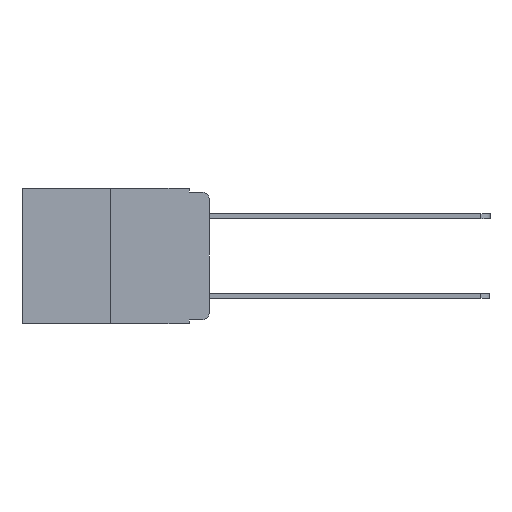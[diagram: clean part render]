
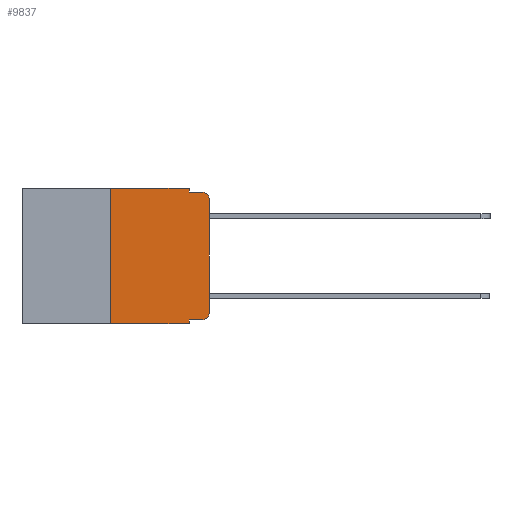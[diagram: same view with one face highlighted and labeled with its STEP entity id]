
A CAD part, left-side view. The second image highlights one B-rep face of the part: STEP entity #9837.
In plain terms, the highlighted planar face has unit normal (-1, 0, 0).
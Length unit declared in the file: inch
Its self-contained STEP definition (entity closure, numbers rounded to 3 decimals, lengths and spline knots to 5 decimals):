
#57 = ORIENTED_EDGE ( 'NONE', *, *, #5798, .T. ) ;
#90 = VERTEX_POINT ( 'NONE', #3340 ) ;
#115 = VERTEX_POINT ( 'NONE', #10934 ) ;
#392 = VECTOR ( 'NONE', #926, 39.37008 ) ;
#569 = VECTOR ( 'NONE', #7066, 39.37008 ) ;
#713 = CARTESIAN_POINT ( 'NONE',  ( 0., 0., -0.03 ) ) ;
#866 = VECTOR ( 'NONE', #9427, 39.37008 ) ;
#926 = DIRECTION ( 'NONE',  ( 0., 0., -1. ) ) ;
#1117 = PLANE ( 'NONE',  #1169 ) ;
#1169 = AXIS2_PLACEMENT_3D ( 'NONE', #7575, #3112, #9108 ) ;
#1266 = ORIENTED_EDGE ( 'NONE', *, *, #5630, .F. ) ;
#1414 = CARTESIAN_POINT ( 'NONE',  ( 0., 0.051, 0. ) ) ;
#1430 = EDGE_CURVE ( 'NONE', #115, #1779, #3272, .T. ) ;
#1488 = ORIENTED_EDGE ( 'NONE', *, *, #1919, .T. ) ;
#1779 = VERTEX_POINT ( 'NONE', #4033 ) ;
#1919 = EDGE_CURVE ( 'NONE', #11219, #90, #7199, .T. ) ;
#1946 = DIRECTION ( 'NONE',  ( -1., 0., 0. ) ) ;
#1982 = VECTOR ( 'NONE', #10357, 39.37008 ) ;
#2005 = DIRECTION ( 'NONE',  ( 0., -1., 0. ) ) ;
#2165 = ORIENTED_EDGE ( 'NONE', *, *, #4709, .F. ) ;
#2188 = VERTEX_POINT ( 'NONE', #1414 ) ;
#2364 = EDGE_CURVE ( 'NONE', #8442, #8231, #5474, .T. ) ;
#2626 = ORIENTED_EDGE ( 'NONE', *, *, #5712, .F. ) ;
#2669 = ORIENTED_EDGE ( 'NONE', *, *, #2364, .T. ) ;
#2711 = FACE_OUTER_BOUND ( 'NONE', #8677, .T. ) ;
#2845 = VERTEX_POINT ( 'NONE', #5978 ) ;
#2976 = VECTOR ( 'NONE', #9016, 39.37008 ) ;
#3112 = DIRECTION ( 'NONE',  ( 1., 0., 0. ) ) ;
#3201 = LINE ( 'NONE', #7888, #866 ) ;
#3229 = ORIENTED_EDGE ( 'NONE', *, *, #5437, .F. ) ;
#3272 = LINE ( 'NONE', #3359, #2976 ) ;
#3340 = CARTESIAN_POINT ( 'NONE',  ( 0., 0., -0.313 ) ) ;
#3341 = VERTEX_POINT ( 'NONE', #8535 ) ;
#3346 = VERTEX_POINT ( 'NONE', #3374 ) ;
#3359 = CARTESIAN_POINT ( 'NONE',  ( 0., 0.473, -0.343 ) ) ;
#3374 = CARTESIAN_POINT ( 'NONE',  ( 0., 0.051, -0.333 ) ) ;
#3418 = LINE ( 'NONE', #9735, #7838 ) ;
#3623 = CARTESIAN_POINT ( 'NONE',  ( 0., 0.051, 0. ) ) ;
#3735 = DIRECTION ( 'NONE',  ( 0., 0., 1. ) ) ;
#3890 = CARTESIAN_POINT ( 'NONE',  ( 0., 0.051, 0. ) ) ;
#4033 = CARTESIAN_POINT ( 'NONE',  ( 0., 0.051, -0.343 ) ) ;
#4662 = ORIENTED_EDGE ( 'NONE', *, *, #1430, .T. ) ;
#4686 = VECTOR ( 'NONE', #2005, 39.37008 ) ;
#4696 = DIRECTION ( 'NONE',  ( -1., 0., 0. ) ) ;
#4709 = EDGE_CURVE ( 'NONE', #3341, #2188, #3418, .T. ) ;
#5263 = AXIS2_PLACEMENT_3D ( 'NONE', #9637, #4696, #10442 ) ;
#5412 = EDGE_CURVE ( 'NONE', #90, #8442, #8141, .T. ) ;
#5437 = EDGE_CURVE ( 'NONE', #2845, #8231, #3201, .T. ) ;
#5474 = CIRCLE ( 'NONE', #8162, 0.02 ) ;
#5485 = CARTESIAN_POINT ( 'NONE',  ( 0., 0.02, -0.01 ) ) ;
#5500 = ORIENTED_EDGE ( 'NONE', *, *, #5767, .F. ) ;
#5590 = LINE ( 'NONE', #3890, #392 ) ;
#5630 = EDGE_CURVE ( 'NONE', #3346, #1779, #7187, .T. ) ;
#5712 = EDGE_CURVE ( 'NONE', #115, #3341, #8489, .T. ) ;
#5767 = EDGE_CURVE ( 'NONE', #2188, #2845, #5590, .T. ) ;
#5798 = EDGE_CURVE ( 'NONE', #3346, #11219, #9856, .T. ) ;
#5837 = CARTESIAN_POINT ( 'NONE',  ( 0., 0.051, -0.333 ) ) ;
#5978 = CARTESIAN_POINT ( 'NONE',  ( 0., 0.051, -0.01 ) ) ;
#6139 = VECTOR ( 'NONE', #3735, 39.37008 ) ;
#7066 = DIRECTION ( 'NONE',  ( 0., 0., 1. ) ) ;
#7187 = LINE ( 'NONE', #3623, #1982 ) ;
#7199 = CIRCLE ( 'NONE', #5263, 0.02 ) ;
#7427 = CARTESIAN_POINT ( 'NONE',  ( 0., 0.02, -0.03 ) ) ;
#7575 = CARTESIAN_POINT ( 'NONE',  ( 0., 0.473, 0. ) ) ;
#7838 = VECTOR ( 'NONE', #10525, 39.37008 ) ;
#7888 = CARTESIAN_POINT ( 'NONE',  ( 0., 0.051, -0.01 ) ) ;
#8141 = LINE ( 'NONE', #8609, #569 ) ;
#8162 = AXIS2_PLACEMENT_3D ( 'NONE', #7427, #1946, #8183 ) ;
#8183 = DIRECTION ( 'NONE',  ( 0., 0., -1. ) ) ;
#8231 = VERTEX_POINT ( 'NONE', #5485 ) ;
#8442 = VERTEX_POINT ( 'NONE', #713 ) ;
#8489 = LINE ( 'NONE', #9643, #6139 ) ;
#8535 = CARTESIAN_POINT ( 'NONE',  ( 0., 0.25, 0. ) ) ;
#8609 = CARTESIAN_POINT ( 'NONE',  ( 0., 0., 0. ) ) ;
#8677 = EDGE_LOOP ( 'NONE', ( #8941, #2669, #3229, #5500, #2165, #2626, #4662, #1266, #57, #1488 ) ) ;
#8941 = ORIENTED_EDGE ( 'NONE', *, *, #5412, .T. ) ;
#9016 = DIRECTION ( 'NONE',  ( 0., -1., 0. ) ) ;
#9018 = CARTESIAN_POINT ( 'NONE',  ( 0., 0.02, -0.333 ) ) ;
#9108 = DIRECTION ( 'NONE',  ( 0., 0., -1. ) ) ;
#9427 = DIRECTION ( 'NONE',  ( 0., -1., 0. ) ) ;
#9637 = CARTESIAN_POINT ( 'NONE',  ( 0., 0.02, -0.313 ) ) ;
#9643 = CARTESIAN_POINT ( 'NONE',  ( 0., 0.25, 0. ) ) ;
#9735 = CARTESIAN_POINT ( 'NONE',  ( 0., 0.473, 0. ) ) ;
#9837 = ADVANCED_FACE ( 'NONE', ( #2711 ), #1117, .F. ) ;
#9856 = LINE ( 'NONE', #5837, #4686 ) ;
#10357 = DIRECTION ( 'NONE',  ( 0., 0., -1. ) ) ;
#10442 = DIRECTION ( 'NONE',  ( 0., 0., -1. ) ) ;
#10525 = DIRECTION ( 'NONE',  ( 0., -1., 0. ) ) ;
#10934 = CARTESIAN_POINT ( 'NONE',  ( 0., 0.25, -0.343 ) ) ;
#11219 = VERTEX_POINT ( 'NONE', #9018 ) ;
